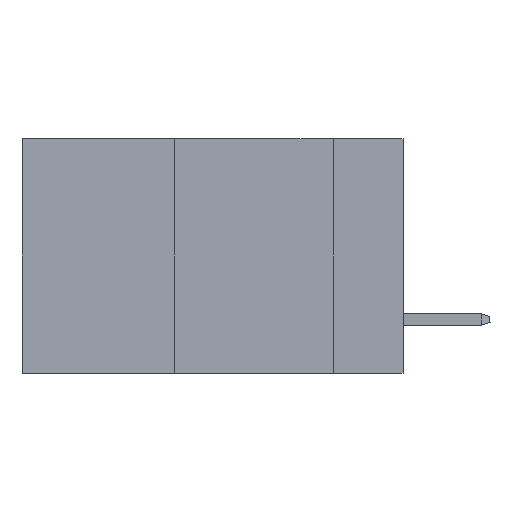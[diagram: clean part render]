
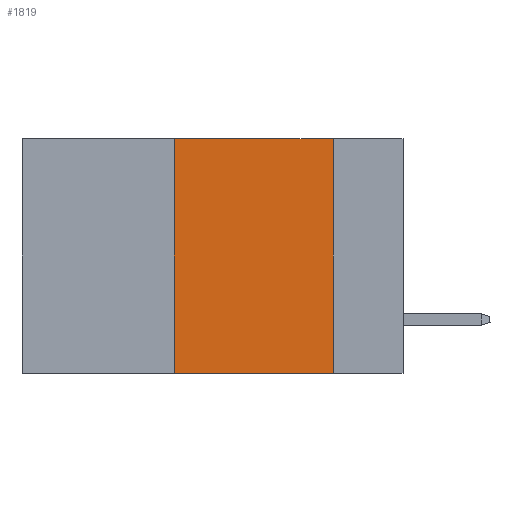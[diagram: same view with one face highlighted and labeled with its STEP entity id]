
A CAD part, left-side view. The second image highlights one B-rep face of the part: STEP entity #1819.
In plain terms, the highlighted planar face has unit normal (-1, 0, 0).
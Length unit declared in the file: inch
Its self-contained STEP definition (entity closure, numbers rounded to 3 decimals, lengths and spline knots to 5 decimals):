
#402 = DIRECTION ( 'NONE',  ( 0., -1., 0. ) ) ;
#1334 = DIRECTION ( 'NONE',  ( 0., 0., -1. ) ) ;
#1482 = EDGE_CURVE ( 'NONE', #15707, #3782, #7832, .T. ) ;
#1819 = ADVANCED_FACE ( 'NONE', ( #14574 ), #4474, .F. ) ;
#2193 = VECTOR ( 'NONE', #402, 39.37008 ) ;
#3452 = DIRECTION ( 'NONE',  ( 0., -1., 0. ) ) ;
#3551 = LINE ( 'NONE', #7858, #8052 ) ;
#3782 = VERTEX_POINT ( 'NONE', #15459 ) ;
#4474 = PLANE ( 'NONE',  #16779 ) ;
#4651 = ORIENTED_EDGE ( 'NONE', *, *, #1482, .T. ) ;
#5120 = EDGE_LOOP ( 'NONE', ( #12688, #12162, #15604, #4651 ) ) ;
#5205 = VERTEX_POINT ( 'NONE', #12546 ) ;
#5239 = LINE ( 'NONE', #9530, #15099 ) ;
#6334 = VERTEX_POINT ( 'NONE', #17631 ) ;
#6428 = CARTESIAN_POINT ( 'NONE',  ( 0., 0.36, -0.37 ) ) ;
#7832 = LINE ( 'NONE', #16670, #2193 ) ;
#7858 = CARTESIAN_POINT ( 'NONE',  ( 0., 0.6, 0. ) ) ;
#8052 = VECTOR ( 'NONE', #3452, 39.37008 ) ;
#8092 = CARTESIAN_POINT ( 'NONE',  ( 0., 0.11, 0. ) ) ;
#8264 = EDGE_CURVE ( 'NONE', #15707, #6334, #5239, .T. ) ;
#8577 = DIRECTION ( 'NONE',  ( 1., 0., 0. ) ) ;
#8672 = CARTESIAN_POINT ( 'NONE',  ( 0., 0.6, 0. ) ) ;
#9530 = CARTESIAN_POINT ( 'NONE',  ( 0., 0.36, 0. ) ) ;
#9816 = LINE ( 'NONE', #8092, #10975 ) ;
#10975 = VECTOR ( 'NONE', #13912, 39.37008 ) ;
#11346 = DIRECTION ( 'NONE',  ( 0., 0., 1. ) ) ;
#12162 = ORIENTED_EDGE ( 'NONE', *, *, #15647, .F. ) ;
#12546 = CARTESIAN_POINT ( 'NONE',  ( 0., 0.11, 0. ) ) ;
#12688 = ORIENTED_EDGE ( 'NONE', *, *, #13494, .F. ) ;
#13494 = EDGE_CURVE ( 'NONE', #5205, #3782, #9816, .T. ) ;
#13912 = DIRECTION ( 'NONE',  ( 0., 0., -1. ) ) ;
#14574 = FACE_OUTER_BOUND ( 'NONE', #5120, .T. ) ;
#15099 = VECTOR ( 'NONE', #11346, 39.37008 ) ;
#15459 = CARTESIAN_POINT ( 'NONE',  ( 0., 0.11, -0.37 ) ) ;
#15604 = ORIENTED_EDGE ( 'NONE', *, *, #8264, .F. ) ;
#15647 = EDGE_CURVE ( 'NONE', #6334, #5205, #3551, .T. ) ;
#15707 = VERTEX_POINT ( 'NONE', #6428 ) ;
#16670 = CARTESIAN_POINT ( 'NONE',  ( 0., 0.6, -0.37 ) ) ;
#16779 = AXIS2_PLACEMENT_3D ( 'NONE', #8672, #8577, #1334 ) ;
#17631 = CARTESIAN_POINT ( 'NONE',  ( 0., 0.36, 0. ) ) ;
